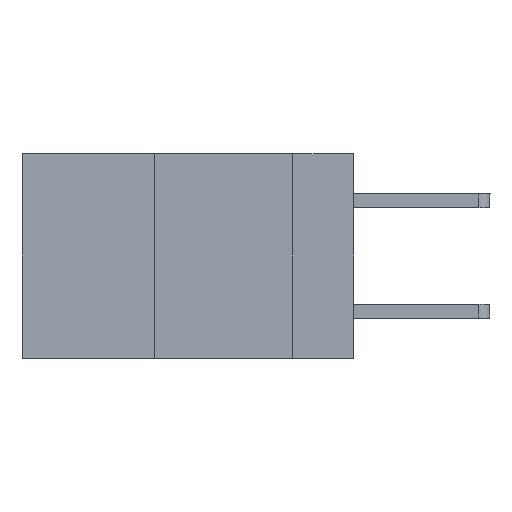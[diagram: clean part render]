
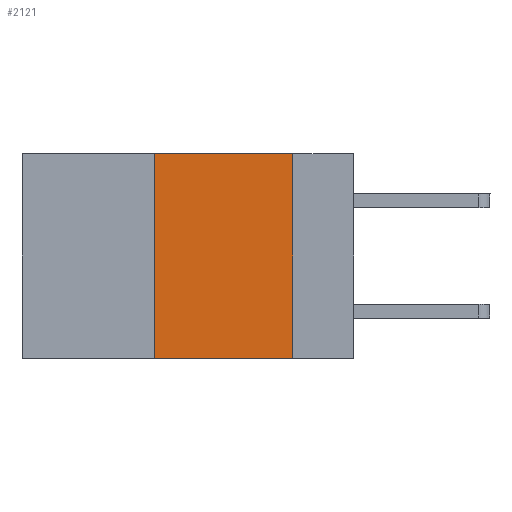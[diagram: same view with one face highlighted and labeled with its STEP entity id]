
A CAD part, left-side view. The second image highlights one B-rep face of the part: STEP entity #2121.
In plain terms, the highlighted planar face has unit normal (-1, 0, 0).
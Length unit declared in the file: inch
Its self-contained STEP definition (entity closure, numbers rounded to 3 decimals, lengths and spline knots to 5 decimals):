
#30 = LINE ( 'NONE', #6880, #6224 ) ;
#693 = ORIENTED_EDGE ( 'NONE', *, *, #10813, .F. ) ;
#814 = DIRECTION ( 'NONE',  ( 0., 0., -1. ) ) ;
#864 = ORIENTED_EDGE ( 'NONE', *, *, #1579, .F. ) ;
#1579 = EDGE_CURVE ( 'NONE', #12247, #4190, #2901, .T. ) ;
#1812 = FACE_OUTER_BOUND ( 'NONE', #7599, .T. ) ;
#2121 = ADVANCED_FACE ( 'NONE', ( #1812 ), #14381, .F. ) ;
#2151 = DIRECTION ( 'NONE',  ( 0., -1., 0. ) ) ;
#2737 = VERTEX_POINT ( 'NONE', #5364 ) ;
#2740 = VECTOR ( 'NONE', #2151, 39.37008 ) ;
#2901 = LINE ( 'NONE', #4260, #14560 ) ;
#3285 = VERTEX_POINT ( 'NONE', #7484 ) ;
#3847 = DIRECTION ( 'NONE',  ( 0., 0., 1. ) ) ;
#4190 = VERTEX_POINT ( 'NONE', #7891 ) ;
#4260 = CARTESIAN_POINT ( 'NONE',  ( 0., 0.11, 0. ) ) ;
#5111 = LINE ( 'NONE', #11800, #13734 ) ;
#5364 = CARTESIAN_POINT ( 'NONE',  ( 0., 0.36, -0.37 ) ) ;
#5392 = DIRECTION ( 'NONE',  ( 0., 0., -1. ) ) ;
#5528 = CARTESIAN_POINT ( 'NONE',  ( 0., 0.11, 0. ) ) ;
#6224 = VECTOR ( 'NONE', #13586, 39.37008 ) ;
#6741 = CARTESIAN_POINT ( 'NONE',  ( 0., 0.6, 0. ) ) ;
#6880 = CARTESIAN_POINT ( 'NONE',  ( 0., 0.6, -0.37 ) ) ;
#7030 = ORIENTED_EDGE ( 'NONE', *, *, #10310, .T. ) ;
#7484 = CARTESIAN_POINT ( 'NONE',  ( 0., 0.36, 0. ) ) ;
#7599 = EDGE_LOOP ( 'NONE', ( #864, #8105, #693, #7030 ) ) ;
#7742 = DIRECTION ( 'NONE',  ( 1., 0., 0. ) ) ;
#7891 = CARTESIAN_POINT ( 'NONE',  ( 0., 0.11, -0.37 ) ) ;
#8105 = ORIENTED_EDGE ( 'NONE', *, *, #11176, .F. ) ;
#9967 = CARTESIAN_POINT ( 'NONE',  ( 0., 0.6, 0. ) ) ;
#10310 = EDGE_CURVE ( 'NONE', #2737, #4190, #30, .T. ) ;
#10813 = EDGE_CURVE ( 'NONE', #2737, #3285, #5111, .T. ) ;
#11176 = EDGE_CURVE ( 'NONE', #3285, #12247, #11856, .T. ) ;
#11800 = CARTESIAN_POINT ( 'NONE',  ( 0., 0.36, 0. ) ) ;
#11856 = LINE ( 'NONE', #6741, #2740 ) ;
#12247 = VERTEX_POINT ( 'NONE', #5528 ) ;
#12545 = AXIS2_PLACEMENT_3D ( 'NONE', #9967, #7742, #814 ) ;
#13586 = DIRECTION ( 'NONE',  ( 0., -1., 0. ) ) ;
#13734 = VECTOR ( 'NONE', #3847, 39.37008 ) ;
#14381 = PLANE ( 'NONE',  #12545 ) ;
#14560 = VECTOR ( 'NONE', #5392, 39.37008 ) ;
